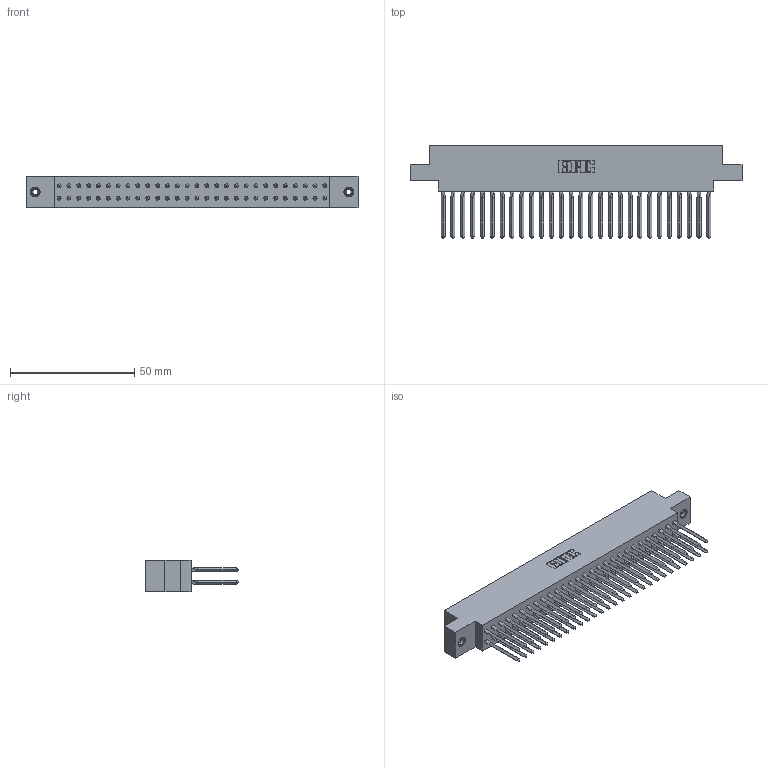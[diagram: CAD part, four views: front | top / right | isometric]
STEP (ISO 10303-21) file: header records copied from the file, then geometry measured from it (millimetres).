
FILE_DESCRIPTION (( 'STEP AP203' ), '1' );
FILE_NAME ('317-056-542-808.STEP', '2020-02-28T04:22:15', ( '' ), ( '' ), 'SwSTEP 2.0', 'SolidWorks 2016', '' );
FILE_SCHEMA (( 'CONFIG_CONTROL_DESIGN' ));
Length unit declared in the file: inch
Products named in the file (4): 345-250-001_345-250-003-102; 317 Part_.156 Dia - TI; 317-056-542-808; 317-290-003_542
Assembly tree (59 placements, depth 2):
  317-056-542-808
    317 Part_.156 Dia - TI
    317-290-003_542  x56
    345-250-001_345-250-003-102  x2
Bounding box: 133.65 x 37.34 x 12.7 mm (x, y, z)
Volume: 21436.6 mm3; surface area: 29382.8 mm2
Topology: 59 solids, 59 shells, 3354 faces, 9371 edges, 5978 vertices
Faces by surface type: plane 2666, cylinder 448, bspline 224, cone 12, torus 4
Entity records: 42630 total; most frequent: CARTESIAN_POINT 7656, ORIENTED_EDGE 7312, DIRECTION 6214, EDGE_CURVE 3656, VECTOR 3466, LINE 3466, VERTEX_POINT 2428, AXIS2_PLACEMENT_3D 1374
